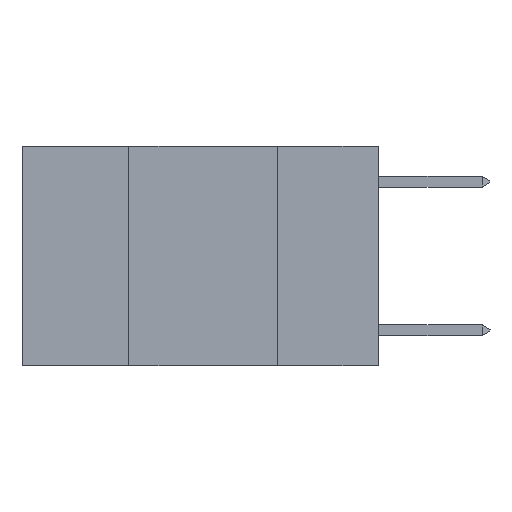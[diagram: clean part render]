
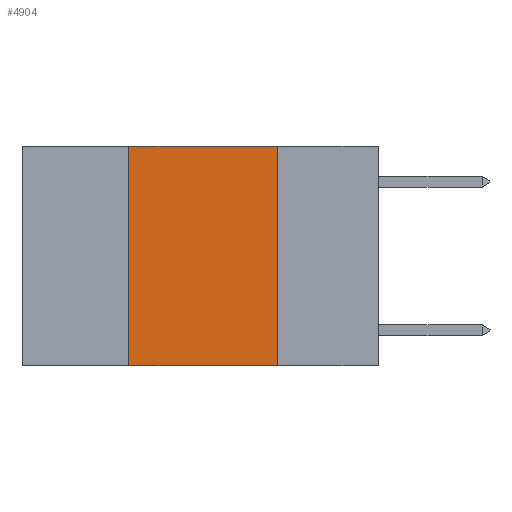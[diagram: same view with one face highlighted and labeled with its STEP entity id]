
A CAD part, left-side view. The second image highlights one B-rep face of the part: STEP entity #4904.
In plain terms, the highlighted planar face has unit normal (-1, 0, 0).
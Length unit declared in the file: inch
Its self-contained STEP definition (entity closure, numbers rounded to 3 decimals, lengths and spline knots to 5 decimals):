
#424 = VERTEX_POINT ( 'NONE', #20967 ) ;
#736 = ORIENTED_EDGE ( 'NONE', *, *, #22012, .T. ) ;
#1511 = CARTESIAN_POINT ( 'NONE',  ( 0., 0.42, 0. ) ) ;
#1776 = PLANE ( 'NONE',  #14230 ) ;
#2336 = ORIENTED_EDGE ( 'NONE', *, *, #5055, .F. ) ;
#2527 = ORIENTED_EDGE ( 'NONE', *, *, #6060, .F. ) ;
#3510 = CARTESIAN_POINT ( 'NONE',  ( 0., 0.17, 0. ) ) ;
#4904 = ADVANCED_FACE ( 'NONE', ( #10411 ), #1776, .F. ) ;
#5045 = CARTESIAN_POINT ( 'NONE',  ( 0., 0.42, 0. ) ) ;
#5055 = EDGE_CURVE ( 'NONE', #29062, #22503, #24725, .T. ) ;
#6060 = EDGE_CURVE ( 'NONE', #22503, #424, #17731, .T. ) ;
#6503 = DIRECTION ( 'NONE',  ( 0., 0., -1. ) ) ;
#7905 = CARTESIAN_POINT ( 'NONE',  ( 0., 0.17, 0. ) ) ;
#9054 = EDGE_LOOP ( 'NONE', ( #2527, #2336, #26777, #736 ) ) ;
#9767 = DIRECTION ( 'NONE',  ( 0., 0., 1. ) ) ;
#10411 = FACE_OUTER_BOUND ( 'NONE', #9054, .T. ) ;
#10626 = DIRECTION ( 'NONE',  ( 0., 0., -1. ) ) ;
#11590 = VECTOR ( 'NONE', #9767, 39.37008 ) ;
#12056 = CARTESIAN_POINT ( 'NONE',  ( 0., 0.42, -0.37 ) ) ;
#12060 = VERTEX_POINT ( 'NONE', #12056 ) ;
#13392 = DIRECTION ( 'NONE',  ( 0., -1., 0. ) ) ;
#14230 = AXIS2_PLACEMENT_3D ( 'NONE', #18268, #20609, #6503 ) ;
#15157 = EDGE_CURVE ( 'NONE', #12060, #29062, #17869, .T. ) ;
#16259 = VECTOR ( 'NONE', #10626, 39.37008 ) ;
#17731 = LINE ( 'NONE', #3510, #16259 ) ;
#17869 = LINE ( 'NONE', #5045, #11590 ) ;
#18268 = CARTESIAN_POINT ( 'NONE',  ( 0., 0.6, 0. ) ) ;
#18400 = VECTOR ( 'NONE', #13392, 39.37008 ) ;
#18518 = VECTOR ( 'NONE', #21112, 39.37008 ) ;
#20609 = DIRECTION ( 'NONE',  ( 1., 0., 0. ) ) ;
#20967 = CARTESIAN_POINT ( 'NONE',  ( 0., 0.17, -0.37 ) ) ;
#21112 = DIRECTION ( 'NONE',  ( 0., -1., 0. ) ) ;
#22012 = EDGE_CURVE ( 'NONE', #12060, #424, #23896, .T. ) ;
#22503 = VERTEX_POINT ( 'NONE', #7905 ) ;
#23896 = LINE ( 'NONE', #27434, #18400 ) ;
#24725 = LINE ( 'NONE', #30395, #18518 ) ;
#26777 = ORIENTED_EDGE ( 'NONE', *, *, #15157, .F. ) ;
#27434 = CARTESIAN_POINT ( 'NONE',  ( 0., 0.6, -0.37 ) ) ;
#29062 = VERTEX_POINT ( 'NONE', #1511 ) ;
#30395 = CARTESIAN_POINT ( 'NONE',  ( 0., 0.6, 0. ) ) ;
